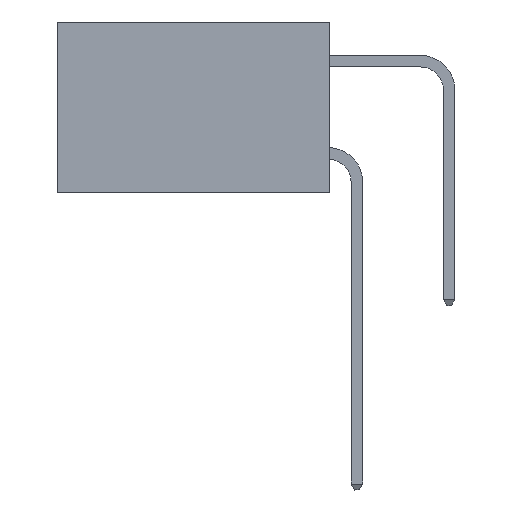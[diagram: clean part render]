
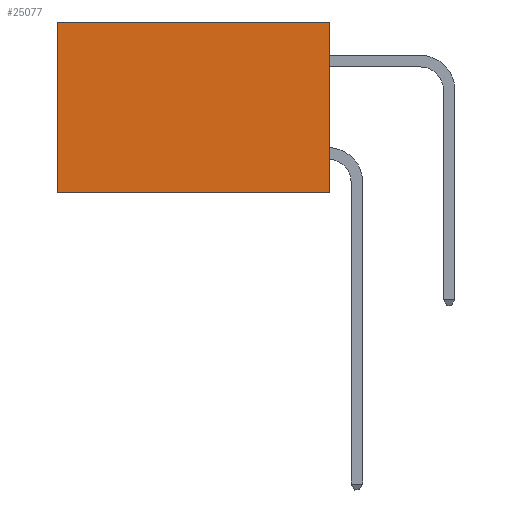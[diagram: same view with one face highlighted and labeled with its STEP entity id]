
A CAD part, left-side view. The second image highlights one B-rep face of the part: STEP entity #25077.
In plain terms, the highlighted planar face has unit normal (-1, 0, 0).
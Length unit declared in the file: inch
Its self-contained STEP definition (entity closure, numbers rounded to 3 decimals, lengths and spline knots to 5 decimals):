
#737 = VECTOR ( 'NONE', #17135, 39.37008 ) ;
#1480 = CARTESIAN_POINT ( 'NONE',  ( 0.277, 0., -0.37 ) ) ;
#1822 = DIRECTION ( 'NONE',  ( 0., 0., -1. ) ) ;
#2752 = ORIENTED_EDGE ( 'NONE', *, *, #21861, .T. ) ;
#3135 = VECTOR ( 'NONE', #11514, 39.37008 ) ;
#5981 = ORIENTED_EDGE ( 'NONE', *, *, #20535, .T. ) ;
#8840 = VERTEX_POINT ( 'NONE', #1480 ) ;
#9538 = ORIENTED_EDGE ( 'NONE', *, *, #24547, .F. ) ;
#10170 = EDGE_LOOP ( 'NONE', ( #2752, #19832, #9538, #5981 ) ) ;
#10800 = VERTEX_POINT ( 'NONE', #22469 ) ;
#10846 = CARTESIAN_POINT ( 'NONE',  ( 0.277, 0., 0. ) ) ;
#10918 = VERTEX_POINT ( 'NONE', #27023 ) ;
#11514 = DIRECTION ( 'NONE',  ( 0., 1., 0. ) ) ;
#13276 = CARTESIAN_POINT ( 'NONE',  ( 0.277, 0.59, -0.37 ) ) ;
#13683 = CARTESIAN_POINT ( 'NONE',  ( 0.277, 0., -0.37 ) ) ;
#14284 = AXIS2_PLACEMENT_3D ( 'NONE', #16923, #14848, #1822 ) ;
#14403 = LINE ( 'NONE', #13276, #18762 ) ;
#14713 = LINE ( 'NONE', #13683, #3135 ) ;
#14848 = DIRECTION ( 'NONE',  ( 1., 0., 0. ) ) ;
#14964 = CARTESIAN_POINT ( 'NONE',  ( 0.277, 0., -0.37 ) ) ;
#15403 = DIRECTION ( 'NONE',  ( 0., 0., -1. ) ) ;
#16750 = EDGE_CURVE ( 'NONE', #8840, #10918, #14713, .T. ) ;
#16923 = CARTESIAN_POINT ( 'NONE',  ( 0.277, 0., -0.37 ) ) ;
#17135 = DIRECTION ( 'NONE',  ( 0., 0., -1. ) ) ;
#18039 = LINE ( 'NONE', #14964, #737 ) ;
#18169 = VECTOR ( 'NONE', #18847, 39.37008 ) ;
#18762 = VECTOR ( 'NONE', #15403, 39.37008 ) ;
#18834 = LINE ( 'NONE', #23075, #18169 ) ;
#18847 = DIRECTION ( 'NONE',  ( 0., 1., 0. ) ) ;
#19832 = ORIENTED_EDGE ( 'NONE', *, *, #16750, .F. ) ;
#20348 = FACE_OUTER_BOUND ( 'NONE', #10170, .T. ) ;
#20535 = EDGE_CURVE ( 'NONE', #21237, #10800, #18834, .T. ) ;
#21237 = VERTEX_POINT ( 'NONE', #10846 ) ;
#21861 = EDGE_CURVE ( 'NONE', #10800, #10918, #14403, .T. ) ;
#22469 = CARTESIAN_POINT ( 'NONE',  ( 0.277, 0.59, 0. ) ) ;
#23075 = CARTESIAN_POINT ( 'NONE',  ( 0.277, 0., 0. ) ) ;
#24547 = EDGE_CURVE ( 'NONE', #21237, #8840, #18039, .T. ) ;
#25077 = ADVANCED_FACE ( 'NONE', ( #20348 ), #27643, .F. ) ;
#27023 = CARTESIAN_POINT ( 'NONE',  ( 0.277, 0.59, -0.37 ) ) ;
#27643 = PLANE ( 'NONE',  #14284 ) ;
